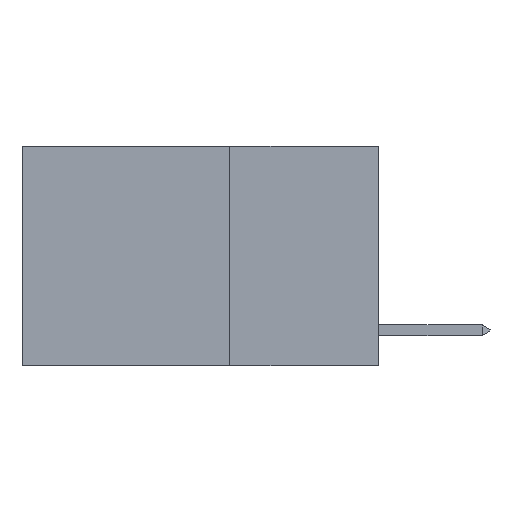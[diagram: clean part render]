
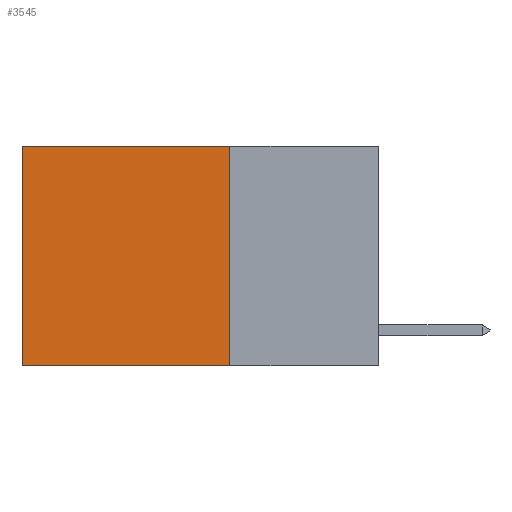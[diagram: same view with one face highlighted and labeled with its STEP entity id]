
A CAD part, left-side view. The second image highlights one B-rep face of the part: STEP entity #3545.
In plain terms, the highlighted planar face has unit normal (-1, 0, 0).
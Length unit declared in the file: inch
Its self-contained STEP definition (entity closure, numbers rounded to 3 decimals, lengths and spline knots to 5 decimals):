
#185 = LINE ( 'NONE', #5307, #11716 ) ;
#1116 = LINE ( 'NONE', #2467, #13932 ) ;
#1824 = ORIENTED_EDGE ( 'NONE', *, *, #8081, .F. ) ;
#2154 = DIRECTION ( 'NONE',  ( 0., 1., 0. ) ) ;
#2467 = CARTESIAN_POINT ( 'NONE',  ( 0.2625, 0.25, -0.37 ) ) ;
#2483 = VERTEX_POINT ( 'NONE', #10450 ) ;
#2832 = CARTESIAN_POINT ( 'NONE',  ( 0.2625, 0.6, -0.37 ) ) ;
#3329 = CARTESIAN_POINT ( 'NONE',  ( 0.2625, 0.25, 0. ) ) ;
#3545 = ADVANCED_FACE ( 'NONE', ( #10210 ), #10760, .F. ) ;
#3993 = CARTESIAN_POINT ( 'NONE',  ( 0.2625, 0.25, 0. ) ) ;
#4641 = VERTEX_POINT ( 'NONE', #2832 ) ;
#4672 = DIRECTION ( 'NONE',  ( 0., 1., 0. ) ) ;
#5028 = DIRECTION ( 'NONE',  ( 0., 0., -1. ) ) ;
#5118 = EDGE_CURVE ( 'NONE', #2483, #4641, #1116, .T. ) ;
#5307 = CARTESIAN_POINT ( 'NONE',  ( 0.2625, 0.6, 0. ) ) ;
#6728 = EDGE_CURVE ( 'NONE', #14031, #4641, #185, .T. ) ;
#6874 = ORIENTED_EDGE ( 'NONE', *, *, #6728, .T. ) ;
#7436 = DIRECTION ( 'NONE',  ( 1., 0., 0. ) ) ;
#7758 = CARTESIAN_POINT ( 'NONE',  ( 0.2625, 0.6, 0. ) ) ;
#8029 = CARTESIAN_POINT ( 'NONE',  ( 0.2625, 0.25, 0. ) ) ;
#8081 = EDGE_CURVE ( 'NONE', #13146, #2483, #12370, .T. ) ;
#8208 = VECTOR ( 'NONE', #2154, 39.37008 ) ;
#9047 = EDGE_LOOP ( 'NONE', ( #6874, #9527, #1824, #10937 ) ) ;
#9347 = VECTOR ( 'NONE', #5028, 39.37008 ) ;
#9527 = ORIENTED_EDGE ( 'NONE', *, *, #5118, .F. ) ;
#10210 = FACE_OUTER_BOUND ( 'NONE', #9047, .T. ) ;
#10450 = CARTESIAN_POINT ( 'NONE',  ( 0.2625, 0.25, -0.37 ) ) ;
#10760 = PLANE ( 'NONE',  #14367 ) ;
#10860 = DIRECTION ( 'NONE',  ( 0., 0., -1. ) ) ;
#10864 = EDGE_CURVE ( 'NONE', #13146, #14031, #14235, .T. ) ;
#10937 = ORIENTED_EDGE ( 'NONE', *, *, #10864, .T. ) ;
#11716 = VECTOR ( 'NONE', #13104, 39.37008 ) ;
#12000 = CARTESIAN_POINT ( 'NONE',  ( 0.2625, 0.25, 0. ) ) ;
#12370 = LINE ( 'NONE', #3993, #9347 ) ;
#13104 = DIRECTION ( 'NONE',  ( 0., 0., -1. ) ) ;
#13146 = VERTEX_POINT ( 'NONE', #8029 ) ;
#13932 = VECTOR ( 'NONE', #4672, 39.37008 ) ;
#14031 = VERTEX_POINT ( 'NONE', #7758 ) ;
#14235 = LINE ( 'NONE', #3329, #8208 ) ;
#14367 = AXIS2_PLACEMENT_3D ( 'NONE', #12000, #7436, #10860 ) ;
